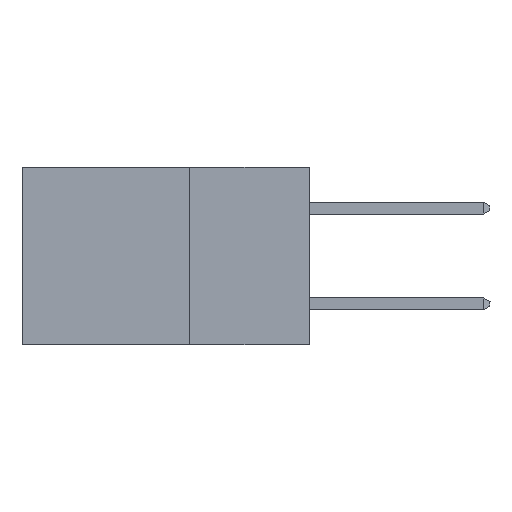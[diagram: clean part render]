
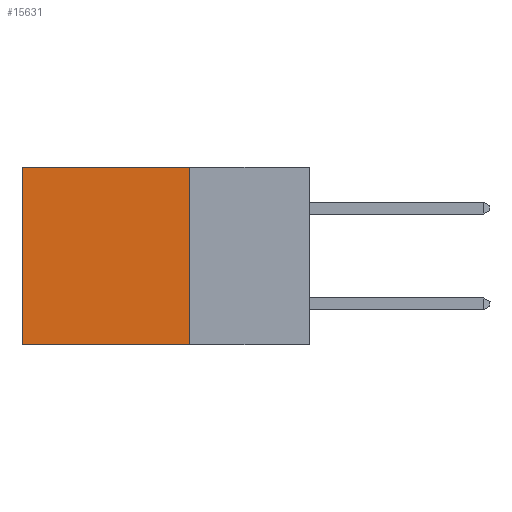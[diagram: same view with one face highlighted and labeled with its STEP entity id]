
A CAD part, left-side view. The second image highlights one B-rep face of the part: STEP entity #15631.
In plain terms, the highlighted planar face has unit normal (-1, 0, 0).
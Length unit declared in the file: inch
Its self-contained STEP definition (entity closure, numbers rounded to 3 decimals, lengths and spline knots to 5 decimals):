
#3316 = CARTESIAN_POINT ( 'NONE',  ( 0.2875, 0.6, -0.37 ) ) ;
#4852 = DIRECTION ( 'NONE',  ( 1., 0., 0. ) ) ;
#5754 = DIRECTION ( 'NONE',  ( 0., 1., 0. ) ) ;
#8806 = LINE ( 'NONE', #32358, #29455 ) ;
#11929 = DIRECTION ( 'NONE',  ( 0., 0., -1. ) ) ;
#13816 = VERTEX_POINT ( 'NONE', #24318 ) ;
#15631 = ADVANCED_FACE ( 'NONE', ( #35907 ), #32480, .F. ) ;
#15981 = VECTOR ( 'NONE', #21172, 39.37008 ) ;
#16701 = CARTESIAN_POINT ( 'NONE',  ( 0.2875, 0.6, 0. ) ) ;
#20059 = EDGE_CURVE ( 'NONE', #28637, #25195, #41833, .T. ) ;
#20133 = CARTESIAN_POINT ( 'NONE',  ( 0.2875, 0.25, 0. ) ) ;
#21172 = DIRECTION ( 'NONE',  ( 0., 1., 0. ) ) ;
#21758 = CARTESIAN_POINT ( 'NONE',  ( 0.2875, 0.25, 0. ) ) ;
#22266 = ORIENTED_EDGE ( 'NONE', *, *, #20059, .T. ) ;
#22729 = DIRECTION ( 'NONE',  ( 0., 0., -1. ) ) ;
#24229 = DIRECTION ( 'NONE',  ( 0., 0., -1. ) ) ;
#24318 = CARTESIAN_POINT ( 'NONE',  ( 0.2875, 0.25, 0. ) ) ;
#25195 = VERTEX_POINT ( 'NONE', #3316 ) ;
#25663 = AXIS2_PLACEMENT_3D ( 'NONE', #21758, #4852, #11929 ) ;
#27493 = EDGE_LOOP ( 'NONE', ( #22266, #43994, #28861, #28342 ) ) ;
#28033 = CARTESIAN_POINT ( 'NONE',  ( 0.2875, 0.25, -0.37 ) ) ;
#28259 = LINE ( 'NONE', #28033, #15981 ) ;
#28342 = ORIENTED_EDGE ( 'NONE', *, *, #44593, .T. ) ;
#28600 = CARTESIAN_POINT ( 'NONE',  ( 0.2875, 0.6, 0. ) ) ;
#28637 = VERTEX_POINT ( 'NONE', #28600 ) ;
#28861 = ORIENTED_EDGE ( 'NONE', *, *, #42226, .F. ) ;
#29455 = VECTOR ( 'NONE', #22729, 39.37008 ) ;
#30291 = VECTOR ( 'NONE', #5754, 39.37008 ) ;
#30642 = LINE ( 'NONE', #20133, #30291 ) ;
#32358 = CARTESIAN_POINT ( 'NONE',  ( 0.2875, 0.25, 0. ) ) ;
#32480 = PLANE ( 'NONE',  #25663 ) ;
#33493 = EDGE_CURVE ( 'NONE', #34945, #25195, #28259, .T. ) ;
#34945 = VERTEX_POINT ( 'NONE', #43570 ) ;
#35907 = FACE_OUTER_BOUND ( 'NONE', #27493, .T. ) ;
#39271 = VECTOR ( 'NONE', #24229, 39.37008 ) ;
#41833 = LINE ( 'NONE', #16701, #39271 ) ;
#42226 = EDGE_CURVE ( 'NONE', #13816, #34945, #8806, .T. ) ;
#43570 = CARTESIAN_POINT ( 'NONE',  ( 0.2875, 0.25, -0.37 ) ) ;
#43994 = ORIENTED_EDGE ( 'NONE', *, *, #33493, .F. ) ;
#44593 = EDGE_CURVE ( 'NONE', #13816, #28637, #30642, .T. ) ;
